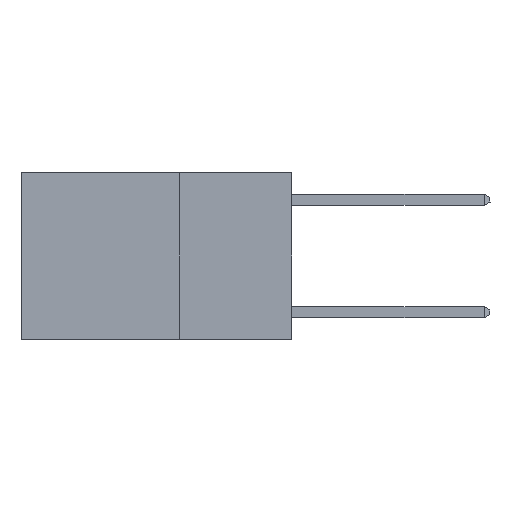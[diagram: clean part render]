
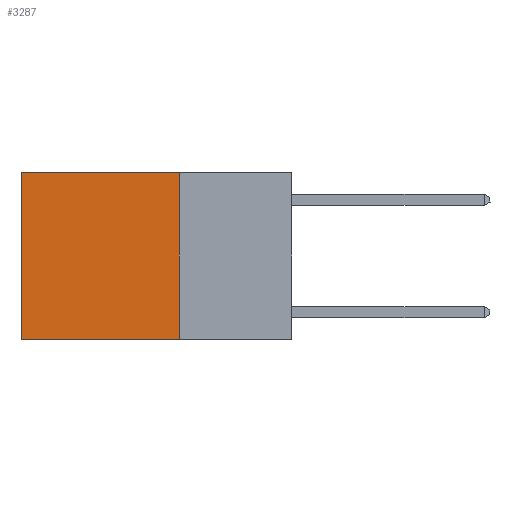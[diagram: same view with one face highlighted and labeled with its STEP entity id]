
A CAD part, left-side view. The second image highlights one B-rep face of the part: STEP entity #3287.
In plain terms, the highlighted planar face has unit normal (-1, 0, 0).
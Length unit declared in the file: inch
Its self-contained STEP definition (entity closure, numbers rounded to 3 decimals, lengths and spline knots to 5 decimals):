
#909 = DIRECTION ( 'NONE',  ( 0., 0., -1. ) ) ;
#1912 = AXIS2_PLACEMENT_3D ( 'NONE', #13961, #15937, #7818 ) ;
#2121 = PLANE ( 'NONE',  #1912 ) ;
#2341 = CARTESIAN_POINT ( 'NONE',  ( 0.2625, 0.25, -0.37 ) ) ;
#2418 = EDGE_CURVE ( 'NONE', #14189, #8997, #7407, .T. ) ;
#2886 = LINE ( 'NONE', #17108, #13926 ) ;
#3287 = ADVANCED_FACE ( 'NONE', ( #24345 ), #2121, .F. ) ;
#4680 = CARTESIAN_POINT ( 'NONE',  ( 0.2625, 0.6, -0.37 ) ) ;
#5117 = ORIENTED_EDGE ( 'NONE', *, *, #19879, .T. ) ;
#5528 = VECTOR ( 'NONE', #19516, 39.37008 ) ;
#5684 = CARTESIAN_POINT ( 'NONE',  ( 0.2625, 0.25, 0. ) ) ;
#6448 = VECTOR ( 'NONE', #909, 39.37008 ) ;
#7209 = EDGE_LOOP ( 'NONE', ( #5117, #10532, #22640, #13020 ) ) ;
#7407 = LINE ( 'NONE', #22167, #5528 ) ;
#7818 = DIRECTION ( 'NONE',  ( 0., 0., -1. ) ) ;
#8899 = EDGE_CURVE ( 'NONE', #8997, #15606, #13460, .T. ) ;
#8997 = VERTEX_POINT ( 'NONE', #2341 ) ;
#10532 = ORIENTED_EDGE ( 'NONE', *, *, #8899, .F. ) ;
#11670 = DIRECTION ( 'NONE',  ( 0., 1., 0. ) ) ;
#13020 = ORIENTED_EDGE ( 'NONE', *, *, #23847, .T. ) ;
#13460 = LINE ( 'NONE', #14000, #20553 ) ;
#13795 = LINE ( 'NONE', #20708, #6448 ) ;
#13926 = VECTOR ( 'NONE', #24995, 39.37008 ) ;
#13961 = CARTESIAN_POINT ( 'NONE',  ( 0.2625, 0.25, 0. ) ) ;
#14000 = CARTESIAN_POINT ( 'NONE',  ( 0.2625, 0.25, -0.37 ) ) ;
#14189 = VERTEX_POINT ( 'NONE', #5684 ) ;
#15606 = VERTEX_POINT ( 'NONE', #4680 ) ;
#15937 = DIRECTION ( 'NONE',  ( 1., 0., 0. ) ) ;
#17108 = CARTESIAN_POINT ( 'NONE',  ( 0.2625, 0.25, 0. ) ) ;
#19516 = DIRECTION ( 'NONE',  ( 0., 0., -1. ) ) ;
#19879 = EDGE_CURVE ( 'NONE', #23932, #15606, #13795, .T. ) ;
#20553 = VECTOR ( 'NONE', #11670, 39.37008 ) ;
#20708 = CARTESIAN_POINT ( 'NONE',  ( 0.2625, 0.6, 0. ) ) ;
#20856 = CARTESIAN_POINT ( 'NONE',  ( 0.2625, 0.6, 0. ) ) ;
#22167 = CARTESIAN_POINT ( 'NONE',  ( 0.2625, 0.25, 0. ) ) ;
#22640 = ORIENTED_EDGE ( 'NONE', *, *, #2418, .F. ) ;
#23847 = EDGE_CURVE ( 'NONE', #14189, #23932, #2886, .T. ) ;
#23932 = VERTEX_POINT ( 'NONE', #20856 ) ;
#24345 = FACE_OUTER_BOUND ( 'NONE', #7209, .T. ) ;
#24995 = DIRECTION ( 'NONE',  ( 0., 1., 0. ) ) ;
